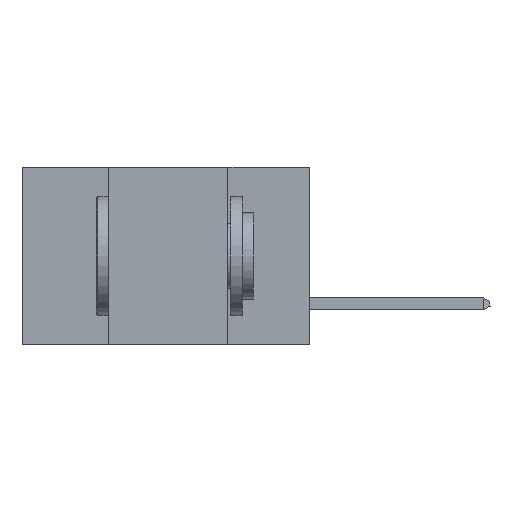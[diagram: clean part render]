
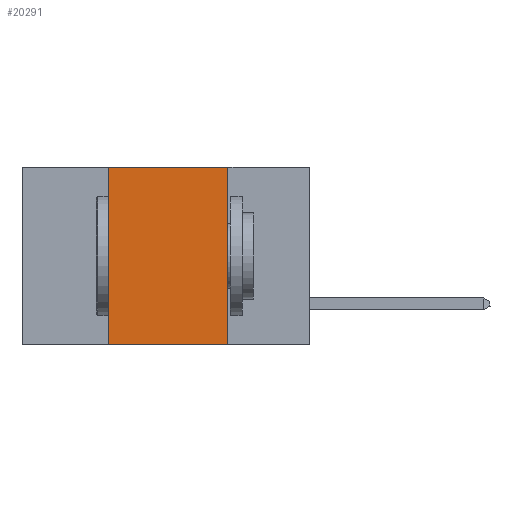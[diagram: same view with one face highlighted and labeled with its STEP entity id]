
A CAD part, left-side view. The second image highlights one B-rep face of the part: STEP entity #20291.
In plain terms, the highlighted planar face has unit normal (-1, 0, 0).
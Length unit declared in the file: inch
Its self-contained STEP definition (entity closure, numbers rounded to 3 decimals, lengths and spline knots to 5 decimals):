
#262 = VECTOR ( 'NONE', #13007, 39.37008 ) ;
#568 = DIRECTION ( 'NONE',  ( 0., 0., -1. ) ) ;
#974 = ORIENTED_EDGE ( 'NONE', *, *, #8508, .F. ) ;
#1125 = CARTESIAN_POINT ( 'NONE',  ( 0., 0.6, 0. ) ) ;
#1646 = VERTEX_POINT ( 'NONE', #7152 ) ;
#1956 = LINE ( 'NONE', #11686, #9696 ) ;
#2353 = CARTESIAN_POINT ( 'NONE',  ( 0., 0.6, -0.37 ) ) ;
#3916 = VECTOR ( 'NONE', #8776, 39.37008 ) ;
#4044 = PLANE ( 'NONE',  #5538 ) ;
#4420 = DIRECTION ( 'NONE',  ( 0., -1., 0. ) ) ;
#4943 = EDGE_CURVE ( 'NONE', #8761, #10613, #8161, .T. ) ;
#5538 = AXIS2_PLACEMENT_3D ( 'NONE', #15199, #16746, #10268 ) ;
#7152 = CARTESIAN_POINT ( 'NONE',  ( 0., 0.17, 0. ) ) ;
#7315 = EDGE_LOOP ( 'NONE', ( #20389, #11688, #974, #11226 ) ) ;
#8161 = LINE ( 'NONE', #2353, #3916 ) ;
#8508 = EDGE_CURVE ( 'NONE', #8761, #17518, #11204, .T. ) ;
#8761 = VERTEX_POINT ( 'NONE', #10667 ) ;
#8776 = DIRECTION ( 'NONE',  ( 0., -1., 0. ) ) ;
#8777 = CARTESIAN_POINT ( 'NONE',  ( 0., 0.17, -0.37 ) ) ;
#9696 = VECTOR ( 'NONE', #568, 39.37008 ) ;
#10268 = DIRECTION ( 'NONE',  ( 0., 0., -1. ) ) ;
#10613 = VERTEX_POINT ( 'NONE', #8777 ) ;
#10667 = CARTESIAN_POINT ( 'NONE',  ( 0., 0.42, -0.37 ) ) ;
#10911 = VECTOR ( 'NONE', #4420, 39.37008 ) ;
#11204 = LINE ( 'NONE', #17811, #262 ) ;
#11226 = ORIENTED_EDGE ( 'NONE', *, *, #4943, .T. ) ;
#11686 = CARTESIAN_POINT ( 'NONE',  ( 0., 0.17, 0. ) ) ;
#11688 = ORIENTED_EDGE ( 'NONE', *, *, #19414, .F. ) ;
#12160 = FACE_OUTER_BOUND ( 'NONE', #7315, .T. ) ;
#12431 = LINE ( 'NONE', #1125, #10911 ) ;
#13007 = DIRECTION ( 'NONE',  ( 0., 0., 1. ) ) ;
#15199 = CARTESIAN_POINT ( 'NONE',  ( 0., 0.6, 0. ) ) ;
#16746 = DIRECTION ( 'NONE',  ( 1., 0., 0. ) ) ;
#17518 = VERTEX_POINT ( 'NONE', #18757 ) ;
#17811 = CARTESIAN_POINT ( 'NONE',  ( 0., 0.42, 0. ) ) ;
#18757 = CARTESIAN_POINT ( 'NONE',  ( 0., 0.42, 0. ) ) ;
#19414 = EDGE_CURVE ( 'NONE', #17518, #1646, #12431, .T. ) ;
#19826 = EDGE_CURVE ( 'NONE', #1646, #10613, #1956, .T. ) ;
#20291 = ADVANCED_FACE ( 'NONE', ( #12160 ), #4044, .F. ) ;
#20389 = ORIENTED_EDGE ( 'NONE', *, *, #19826, .F. ) ;
